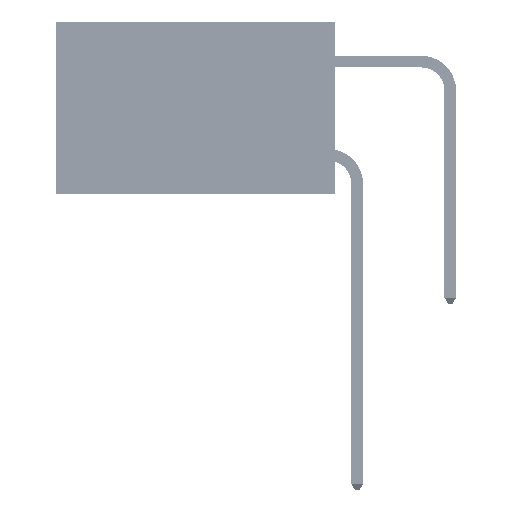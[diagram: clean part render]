
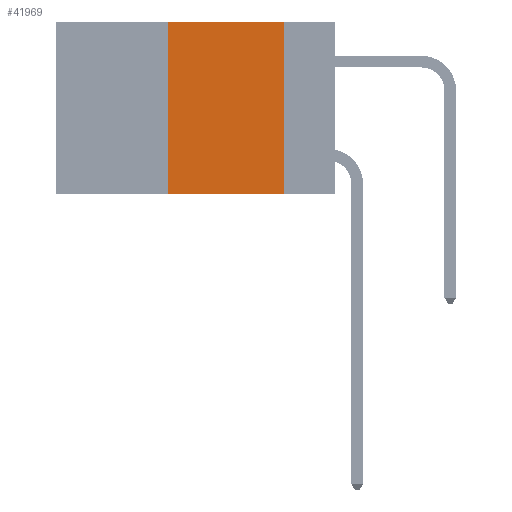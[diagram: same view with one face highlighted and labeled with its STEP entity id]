
A CAD part, left-side view. The second image highlights one B-rep face of the part: STEP entity #41969.
In plain terms, the highlighted planar face has unit normal (-1, 0, 0).
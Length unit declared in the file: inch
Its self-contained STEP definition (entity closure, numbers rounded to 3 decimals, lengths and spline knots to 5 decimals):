
#1857 = EDGE_CURVE ( 'NONE', #37734, #19003, #27726, .T. ) ;
#2519 = PLANE ( 'NONE',  #42660 ) ;
#4778 = DIRECTION ( 'NONE',  ( 0., 0., 1. ) ) ;
#4951 = VECTOR ( 'NONE', #29117, 39.37008 ) ;
#5619 = CARTESIAN_POINT ( 'NONE',  ( 0., 0.36, -0.37 ) ) ;
#7293 = CARTESIAN_POINT ( 'NONE',  ( 0., 0.6, 0. ) ) ;
#9405 = CARTESIAN_POINT ( 'NONE',  ( 0., 0.11, 0. ) ) ;
#9877 = CARTESIAN_POINT ( 'NONE',  ( 0., 0.6, 0. ) ) ;
#11930 = EDGE_CURVE ( 'NONE', #37734, #44679, #40297, .T. ) ;
#12420 = VECTOR ( 'NONE', #32397, 39.37008 ) ;
#12666 = VECTOR ( 'NONE', #38492, 39.37008 ) ;
#14094 = CARTESIAN_POINT ( 'NONE',  ( 0., 0.11, -0.37 ) ) ;
#14639 = LINE ( 'NONE', #7293, #4951 ) ;
#17940 = CARTESIAN_POINT ( 'NONE',  ( 0., 0.6, -0.37 ) ) ;
#19003 = VERTEX_POINT ( 'NONE', #29161 ) ;
#19717 = FACE_OUTER_BOUND ( 'NONE', #31005, .T. ) ;
#20865 = DIRECTION ( 'NONE',  ( 1., 0., 0. ) ) ;
#22491 = ORIENTED_EDGE ( 'NONE', *, *, #23532, .F. ) ;
#22612 = CARTESIAN_POINT ( 'NONE',  ( 0., 0.11, 0. ) ) ;
#23532 = EDGE_CURVE ( 'NONE', #23836, #44679, #32075, .T. ) ;
#23836 = VERTEX_POINT ( 'NONE', #22612 ) ;
#24757 = ORIENTED_EDGE ( 'NONE', *, *, #11930, .T. ) ;
#27726 = LINE ( 'NONE', #30280, #45828 ) ;
#29117 = DIRECTION ( 'NONE',  ( 0., -1., 0. ) ) ;
#29161 = CARTESIAN_POINT ( 'NONE',  ( 0., 0.36, 0. ) ) ;
#30280 = CARTESIAN_POINT ( 'NONE',  ( 0., 0.36, 0. ) ) ;
#31005 = EDGE_LOOP ( 'NONE', ( #22491, #36699, #40534, #24757 ) ) ;
#32075 = LINE ( 'NONE', #9405, #12666 ) ;
#32397 = DIRECTION ( 'NONE',  ( 0., -1., 0. ) ) ;
#34857 = EDGE_CURVE ( 'NONE', #19003, #23836, #14639, .T. ) ;
#36699 = ORIENTED_EDGE ( 'NONE', *, *, #34857, .F. ) ;
#37734 = VERTEX_POINT ( 'NONE', #5619 ) ;
#38492 = DIRECTION ( 'NONE',  ( 0., 0., -1. ) ) ;
#40297 = LINE ( 'NONE', #17940, #12420 ) ;
#40534 = ORIENTED_EDGE ( 'NONE', *, *, #1857, .F. ) ;
#41969 = ADVANCED_FACE ( 'NONE', ( #19717 ), #2519, .F. ) ;
#42660 = AXIS2_PLACEMENT_3D ( 'NONE', #9877, #20865, #46217 ) ;
#44679 = VERTEX_POINT ( 'NONE', #14094 ) ;
#45828 = VECTOR ( 'NONE', #4778, 39.37008 ) ;
#46217 = DIRECTION ( 'NONE',  ( 0., 0., -1. ) ) ;
